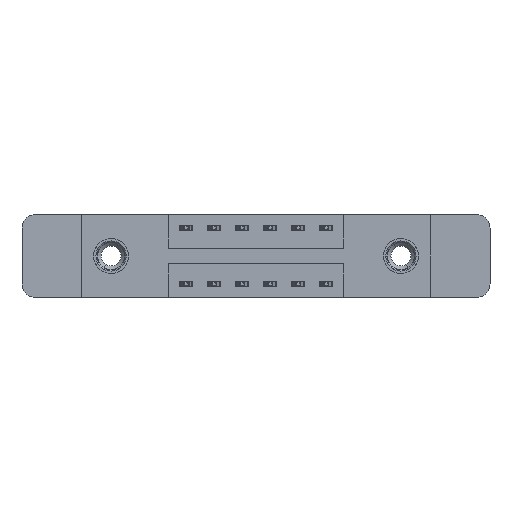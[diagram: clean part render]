
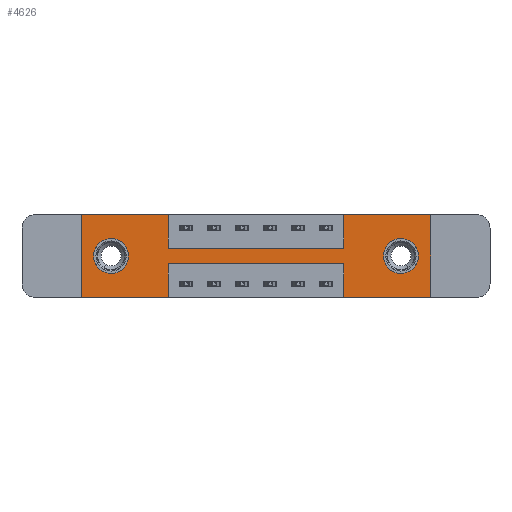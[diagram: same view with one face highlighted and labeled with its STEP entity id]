
A CAD part, front view. The second image highlights one B-rep face of the part: STEP entity #4626.
In plain terms, the highlighted planar face has unit normal (0, -1, 0).
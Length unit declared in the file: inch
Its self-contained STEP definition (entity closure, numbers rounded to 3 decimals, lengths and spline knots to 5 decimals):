
#53 = CARTESIAN_POINT ( 'NONE',  ( 0., 0., 0. ) ) ;
#78 = LINE ( 'NONE', #3523, #10589 ) ;
#163 = CARTESIAN_POINT ( 'NONE',  ( 0.3875, 0., -0.15 ) ) ;
#217 = CARTESIAN_POINT ( 'NONE',  ( 1.1725, 0., 0. ) ) ;
#222 = EDGE_CURVE ( 'NONE', #9883, #817, #8737, .T. ) ;
#253 = LINE ( 'NONE', #6098, #13097 ) ;
#377 = EDGE_CURVE ( 'NONE', #3911, #12588, #13431, .T. ) ;
#395 = CARTESIAN_POINT ( 'NONE',  ( 0.3875, 0., -0.22 ) ) ;
#411 = VERTEX_POINT ( 'NONE', #7562 ) ;
#419 = CARTESIAN_POINT ( 'NONE',  ( 1.1725, 0., -0.37 ) ) ;
#461 = EDGE_CURVE ( 'NONE', #6841, #12114, #10743, .T. ) ;
#468 = FACE_OUTER_BOUND ( 'NONE', #803, .T. ) ;
#762 = ORIENTED_EDGE ( 'NONE', *, *, #11061, .T. ) ;
#803 = EDGE_LOOP ( 'NONE', ( #3731, #9505, #13849, #3143, #1140, #6147, #10958, #9661, #5859, #11640, #12063, #2747 ) ) ;
#817 = VERTEX_POINT ( 'NONE', #11268 ) ;
#912 = EDGE_CURVE ( 'NONE', #411, #8628, #4987, .T. ) ;
#918 = AXIS2_PLACEMENT_3D ( 'NONE', #7209, #4161, #973 ) ;
#973 = DIRECTION ( 'NONE',  ( 0., 0., 1. ) ) ;
#1068 = ORIENTED_EDGE ( 'NONE', *, *, #12971, .T. ) ;
#1140 = ORIENTED_EDGE ( 'NONE', *, *, #2922, .F. ) ;
#1196 = DIRECTION ( 'NONE',  ( 0., 0., 1. ) ) ;
#1340 = LINE ( 'NONE', #7072, #12519 ) ;
#1442 = DIRECTION ( 'NONE',  ( 0., 0., -1. ) ) ;
#1461 = CARTESIAN_POINT ( 'NONE',  ( 1.1725, 0., -0.37 ) ) ;
#1680 = DIRECTION ( 'NONE',  ( 0., 0., -1. ) ) ;
#1742 = VERTEX_POINT ( 'NONE', #163 ) ;
#1789 = EDGE_CURVE ( 'NONE', #7474, #1742, #1340, .T. ) ;
#2500 = DIRECTION ( 'NONE',  ( -1., 0., 0. ) ) ;
#2574 = CARTESIAN_POINT ( 'NONE',  ( 0.3875, 0., -0.22 ) ) ;
#2684 = DIRECTION ( 'NONE',  ( 0., 0., 1. ) ) ;
#2689 = CARTESIAN_POINT ( 'NONE',  ( 0., 0., -0.37 ) ) ;
#2747 = ORIENTED_EDGE ( 'NONE', *, *, #13048, .F. ) ;
#2922 = EDGE_CURVE ( 'NONE', #9874, #5498, #10400, .T. ) ;
#3121 = VERTEX_POINT ( 'NONE', #1461 ) ;
#3125 = LINE ( 'NONE', #53, #9532 ) ;
#3143 = ORIENTED_EDGE ( 'NONE', *, *, #7777, .F. ) ;
#3369 = EDGE_CURVE ( 'NONE', #12114, #9874, #4257, .T. ) ;
#3523 = CARTESIAN_POINT ( 'NONE',  ( 0., 0., -0.37 ) ) ;
#3568 = CARTESIAN_POINT ( 'NONE',  ( 1.4275, 0., -0.185 ) ) ;
#3619 = CARTESIAN_POINT ( 'NONE',  ( 0., 0., -0.37 ) ) ;
#3656 = DIRECTION ( 'NONE',  ( -1., 0., 0. ) ) ;
#3731 = ORIENTED_EDGE ( 'NONE', *, *, #12100, .F. ) ;
#3759 = DIRECTION ( 'NONE',  ( 0., 0., -1. ) ) ;
#3846 = CARTESIAN_POINT ( 'NONE',  ( 1.4275, 0., -0.263 ) ) ;
#3911 = VERTEX_POINT ( 'NONE', #10458 ) ;
#3920 = AXIS2_PLACEMENT_3D ( 'NONE', #8229, #9319, #1680 ) ;
#4151 = ORIENTED_EDGE ( 'NONE', *, *, #9889, .T. ) ;
#4161 = DIRECTION ( 'NONE',  ( 0., 1., 0. ) ) ;
#4231 = LINE ( 'NONE', #419, #7100 ) ;
#4257 = LINE ( 'NONE', #10456, #13207 ) ;
#4356 = CIRCLE ( 'NONE', #918, 0.078 ) ;
#4438 = CARTESIAN_POINT ( 'NONE',  ( 0.1325, 0., -0.185 ) ) ;
#4626 = ADVANCED_FACE ( 'NONE', ( #5367, #12668, #468 ), #9347, .T. ) ;
#4987 = LINE ( 'NONE', #2574, #13407 ) ;
#5068 = LINE ( 'NONE', #7923, #13482 ) ;
#5168 = EDGE_CURVE ( 'NONE', #1742, #6841, #5068, .T. ) ;
#5287 = VECTOR ( 'NONE', #8826, 39.37008 ) ;
#5367 = FACE_BOUND ( 'NONE', #6382, .T. ) ;
#5498 = VERTEX_POINT ( 'NONE', #9111 ) ;
#5779 = VERTEX_POINT ( 'NONE', #10433 ) ;
#5859 = ORIENTED_EDGE ( 'NONE', *, *, #1789, .F. ) ;
#6009 = DIRECTION ( 'NONE',  ( 0., -1., 0. ) ) ;
#6094 = EDGE_LOOP ( 'NONE', ( #12090, #762 ) ) ;
#6098 = CARTESIAN_POINT ( 'NONE',  ( 0.3875, 0., -0.37 ) ) ;
#6147 = ORIENTED_EDGE ( 'NONE', *, *, #3369, .F. ) ;
#6204 = DIRECTION ( 'NONE',  ( 0., 0., -1. ) ) ;
#6382 = EDGE_LOOP ( 'NONE', ( #1068, #4151 ) ) ;
#6841 = VERTEX_POINT ( 'NONE', #7416 ) ;
#7072 = CARTESIAN_POINT ( 'NONE',  ( 0.3875, 0., 0. ) ) ;
#7092 = AXIS2_PLACEMENT_3D ( 'NONE', #2689, #6009, #11454 ) ;
#7100 = VECTOR ( 'NONE', #2684, 39.37008 ) ;
#7199 = VECTOR ( 'NONE', #1196, 39.37008 ) ;
#7209 = CARTESIAN_POINT ( 'NONE',  ( 0.1325, 0., -0.185 ) ) ;
#7405 = CARTESIAN_POINT ( 'NONE',  ( 0.3875, 0., 0. ) ) ;
#7413 = DIRECTION ( 'NONE',  ( 0., 0., 1. ) ) ;
#7416 = CARTESIAN_POINT ( 'NONE',  ( 1.1725, 0., -0.15 ) ) ;
#7440 = CARTESIAN_POINT ( 'NONE',  ( 0.3875, 0., -0.37 ) ) ;
#7474 = VERTEX_POINT ( 'NONE', #7405 ) ;
#7518 = CARTESIAN_POINT ( 'NONE',  ( 0., 0., 0. ) ) ;
#7562 = CARTESIAN_POINT ( 'NONE',  ( 1.1725, 0., -0.22 ) ) ;
#7777 = EDGE_CURVE ( 'NONE', #5498, #3121, #12406, .T. ) ;
#7780 = CARTESIAN_POINT ( 'NONE',  ( 1.56, 0., 0. ) ) ;
#7923 = CARTESIAN_POINT ( 'NONE',  ( 0.3875, 0., -0.15 ) ) ;
#8068 = EDGE_CURVE ( 'NONE', #12588, #7474, #3125, .T. ) ;
#8229 = CARTESIAN_POINT ( 'NONE',  ( 1.4275, 0., -0.185 ) ) ;
#8628 = VERTEX_POINT ( 'NONE', #395 ) ;
#8737 = CIRCLE ( 'NONE', #10908, 0.078 ) ;
#8807 = VERTEX_POINT ( 'NONE', #7440 ) ;
#8826 = DIRECTION ( 'NONE',  ( 0., 0., -1. ) ) ;
#8853 = DIRECTION ( 'NONE',  ( 1., 0., 0. ) ) ;
#9111 = CARTESIAN_POINT ( 'NONE',  ( 1.56, 0., -0.37 ) ) ;
#9319 = DIRECTION ( 'NONE',  ( 0., 1., 0. ) ) ;
#9347 = PLANE ( 'NONE',  #7092 ) ;
#9505 = ORIENTED_EDGE ( 'NONE', *, *, #912, .F. ) ;
#9532 = VECTOR ( 'NONE', #8853, 39.37008 ) ;
#9549 = VECTOR ( 'NONE', #2500, 39.37008 ) ;
#9563 = CIRCLE ( 'NONE', #13329, 0.078 ) ;
#9661 = ORIENTED_EDGE ( 'NONE', *, *, #5168, .F. ) ;
#9779 = EDGE_CURVE ( 'NONE', #3121, #411, #4231, .T. ) ;
#9874 = VERTEX_POINT ( 'NONE', #10370 ) ;
#9883 = VERTEX_POINT ( 'NONE', #12476 ) ;
#9889 = EDGE_CURVE ( 'NONE', #11832, #5779, #12158, .T. ) ;
#9983 = CARTESIAN_POINT ( 'NONE',  ( 0., 0., 0. ) ) ;
#10155 = DIRECTION ( 'NONE',  ( 0., 1., 0. ) ) ;
#10370 = CARTESIAN_POINT ( 'NONE',  ( 1.56, 0., 0. ) ) ;
#10400 = LINE ( 'NONE', #7780, #5287 ) ;
#10433 = CARTESIAN_POINT ( 'NONE',  ( 1.4275, 0., -0.107 ) ) ;
#10456 = CARTESIAN_POINT ( 'NONE',  ( 0., 0., 0. ) ) ;
#10458 = CARTESIAN_POINT ( 'NONE',  ( 0., 0., -0.37 ) ) ;
#10589 = VECTOR ( 'NONE', #11091, 39.37008 ) ;
#10633 = DIRECTION ( 'NONE',  ( 0., 1., 0. ) ) ;
#10743 = LINE ( 'NONE', #217, #7199 ) ;
#10908 = AXIS2_PLACEMENT_3D ( 'NONE', #4438, #10633, #13025 ) ;
#10958 = ORIENTED_EDGE ( 'NONE', *, *, #461, .F. ) ;
#11061 = EDGE_CURVE ( 'NONE', #817, #9883, #4356, .T. ) ;
#11091 = DIRECTION ( 'NONE',  ( -1., 0., 0. ) ) ;
#11268 = CARTESIAN_POINT ( 'NONE',  ( 0.1325, 0., -0.263 ) ) ;
#11454 = DIRECTION ( 'NONE',  ( 0., 0., -1. ) ) ;
#11640 = ORIENTED_EDGE ( 'NONE', *, *, #8068, .F. ) ;
#11832 = VERTEX_POINT ( 'NONE', #3846 ) ;
#12063 = ORIENTED_EDGE ( 'NONE', *, *, #377, .F. ) ;
#12090 = ORIENTED_EDGE ( 'NONE', *, *, #222, .T. ) ;
#12100 = EDGE_CURVE ( 'NONE', #8628, #8807, #253, .T. ) ;
#12114 = VERTEX_POINT ( 'NONE', #12636 ) ;
#12158 = CIRCLE ( 'NONE', #3920, 0.078 ) ;
#12406 = LINE ( 'NONE', #3619, #9549 ) ;
#12476 = CARTESIAN_POINT ( 'NONE',  ( 0.1325, 0., -0.107 ) ) ;
#12519 = VECTOR ( 'NONE', #3759, 39.37008 ) ;
#12568 = DIRECTION ( 'NONE',  ( 1., 0., 0. ) ) ;
#12588 = VERTEX_POINT ( 'NONE', #9983 ) ;
#12636 = CARTESIAN_POINT ( 'NONE',  ( 1.1725, 0., 0. ) ) ;
#12668 = FACE_BOUND ( 'NONE', #6094, .T. ) ;
#12971 = EDGE_CURVE ( 'NONE', #5779, #11832, #9563, .T. ) ;
#13025 = DIRECTION ( 'NONE',  ( 0., 0., 1. ) ) ;
#13048 = EDGE_CURVE ( 'NONE', #8807, #3911, #78, .T. ) ;
#13097 = VECTOR ( 'NONE', #6204, 39.37008 ) ;
#13207 = VECTOR ( 'NONE', #13620, 39.37008 ) ;
#13329 = AXIS2_PLACEMENT_3D ( 'NONE', #3568, #10155, #1442 ) ;
#13407 = VECTOR ( 'NONE', #3656, 39.37008 ) ;
#13431 = LINE ( 'NONE', #7518, #13945 ) ;
#13482 = VECTOR ( 'NONE', #12568, 39.37008 ) ;
#13620 = DIRECTION ( 'NONE',  ( 1., 0., 0. ) ) ;
#13849 = ORIENTED_EDGE ( 'NONE', *, *, #9779, .F. ) ;
#13945 = VECTOR ( 'NONE', #7413, 39.37008 ) ;
